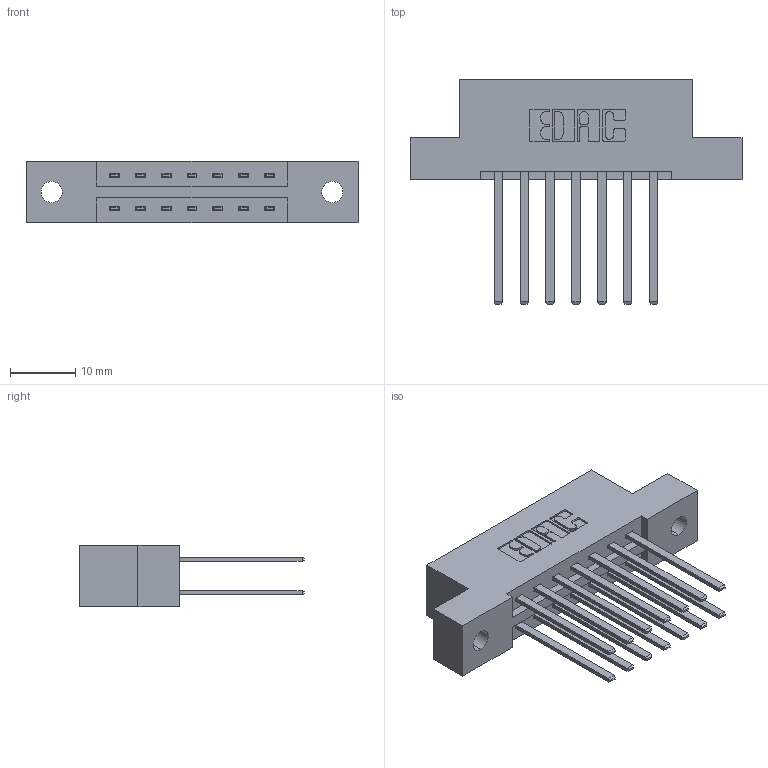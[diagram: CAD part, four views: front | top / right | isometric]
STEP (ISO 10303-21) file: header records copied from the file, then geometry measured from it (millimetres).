
FILE_DESCRIPTION (( 'STEP AP203' ), '1' );
FILE_NAME ('337-014-544-202.STEP', '2019-10-08T11:51:25', ( '' ), ( '' ), 'SwSTEP 2.0', 'SolidWorks 2016', '' );
FILE_SCHEMA (( 'CONFIG_CONTROL_DESIGN' ));
Length unit declared in the file: inch
Products named in the file (3): 345-292-001_345-293-144; 337 Part_Flush Mounting Lugs - 0.128 Dia; 337-014-544-202
Assembly tree (15 placements, depth 2):
  337-014-544-202
    337 Part_Flush Mounting Lugs - 0.128 Dia
    345-292-001_345-293-144  x14
Bounding box: 50.75 x 34.3 x 9.4 mm (x, y, z)
Volume: 5042 mm3; surface area: 5728.5 mm2
Topology: 15 solids, 15 shells, 786 faces, 2313 edges, 1522 vertices
Faces by surface type: plane 546, cylinder 240
Entity records: 9773 total; most frequent: CARTESIAN_POINT 1674, ORIENTED_EDGE 1610, DIRECTION 1485, EDGE_CURVE 805, VECTOR 681, LINE 681, VERTEX_POINT 534, AXIS2_PLACEMENT_3D 402
